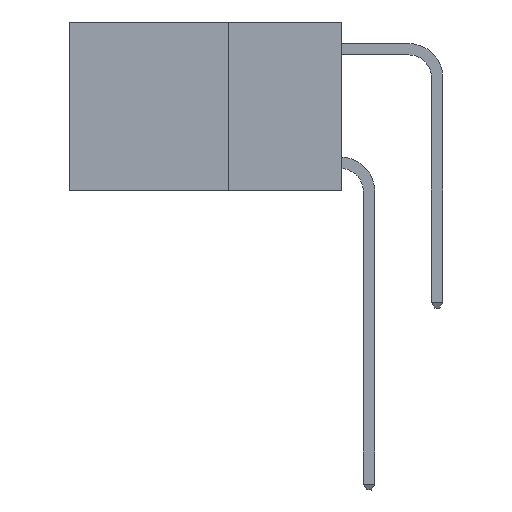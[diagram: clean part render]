
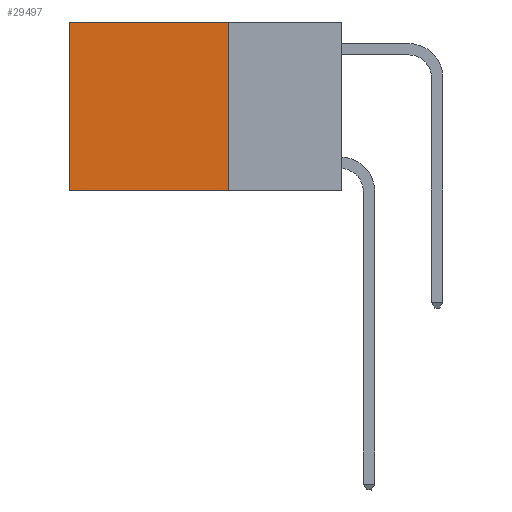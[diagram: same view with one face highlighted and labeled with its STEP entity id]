
A CAD part, left-side view. The second image highlights one B-rep face of the part: STEP entity #29497.
In plain terms, the highlighted planar face has unit normal (-1, 0, 0).
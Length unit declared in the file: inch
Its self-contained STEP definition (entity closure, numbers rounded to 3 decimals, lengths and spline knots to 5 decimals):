
#60 = DIRECTION ( 'NONE',  ( 0., 0., -1. ) ) ;
#1233 = ORIENTED_EDGE ( 'NONE', *, *, #20882, .F. ) ;
#1363 = AXIS2_PLACEMENT_3D ( 'NONE', #8261, #26635, #12900 ) ;
#5061 = CARTESIAN_POINT ( 'NONE',  ( 0.2625, 0.6, 0. ) ) ;
#5254 = VERTEX_POINT ( 'NONE', #18942 ) ;
#6689 = VERTEX_POINT ( 'NONE', #19164 ) ;
#7974 = CARTESIAN_POINT ( 'NONE',  ( 0.2625, 0.25, 0. ) ) ;
#8261 = CARTESIAN_POINT ( 'NONE',  ( 0.2625, 0.25, 0. ) ) ;
#8386 = CARTESIAN_POINT ( 'NONE',  ( 0.2625, 0.25, -0.37 ) ) ;
#10280 = DIRECTION ( 'NONE',  ( 0., 0., -1. ) ) ;
#10582 = PLANE ( 'NONE',  #1363 ) ;
#10790 = LINE ( 'NONE', #13990, #28391 ) ;
#12900 = DIRECTION ( 'NONE',  ( 0., 0., -1. ) ) ;
#13990 = CARTESIAN_POINT ( 'NONE',  ( 0.2625, 0.6, 0. ) ) ;
#14975 = VECTOR ( 'NONE', #17416, 39.37008 ) ;
#15669 = FACE_OUTER_BOUND ( 'NONE', #26213, .T. ) ;
#16015 = EDGE_CURVE ( 'NONE', #18665, #5254, #17664, .T. ) ;
#17416 = DIRECTION ( 'NONE',  ( 0., 1., 0. ) ) ;
#17486 = VECTOR ( 'NONE', #22138, 39.37008 ) ;
#17664 = LINE ( 'NONE', #7974, #29156 ) ;
#18665 = VERTEX_POINT ( 'NONE', #22589 ) ;
#18942 = CARTESIAN_POINT ( 'NONE',  ( 0.2625, 0.25, -0.37 ) ) ;
#19164 = CARTESIAN_POINT ( 'NONE',  ( 0.2625, 0.6, -0.37 ) ) ;
#19502 = ORIENTED_EDGE ( 'NONE', *, *, #29476, .T. ) ;
#20882 = EDGE_CURVE ( 'NONE', #5254, #6689, #29686, .T. ) ;
#22138 = DIRECTION ( 'NONE',  ( 0., 1., 0. ) ) ;
#22589 = CARTESIAN_POINT ( 'NONE',  ( 0.2625, 0.25, 0. ) ) ;
#23281 = ORIENTED_EDGE ( 'NONE', *, *, #24761, .T. ) ;
#24236 = CARTESIAN_POINT ( 'NONE',  ( 0.2625, 0.25, 0. ) ) ;
#24761 = EDGE_CURVE ( 'NONE', #26541, #6689, #10790, .T. ) ;
#26213 = EDGE_LOOP ( 'NONE', ( #23281, #1233, #29738, #19502 ) ) ;
#26541 = VERTEX_POINT ( 'NONE', #5061 ) ;
#26635 = DIRECTION ( 'NONE',  ( 1., 0., 0. ) ) ;
#27148 = LINE ( 'NONE', #24236, #14975 ) ;
#28391 = VECTOR ( 'NONE', #60, 39.37008 ) ;
#29156 = VECTOR ( 'NONE', #10280, 39.37008 ) ;
#29476 = EDGE_CURVE ( 'NONE', #18665, #26541, #27148, .T. ) ;
#29497 = ADVANCED_FACE ( 'NONE', ( #15669 ), #10582, .F. ) ;
#29686 = LINE ( 'NONE', #8386, #17486 ) ;
#29738 = ORIENTED_EDGE ( 'NONE', *, *, #16015, .F. ) ;
